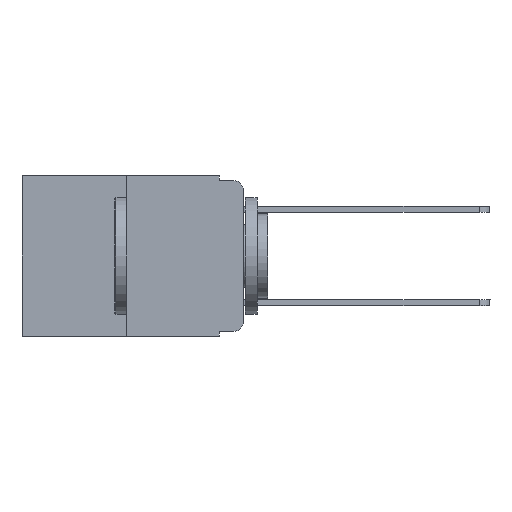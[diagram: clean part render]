
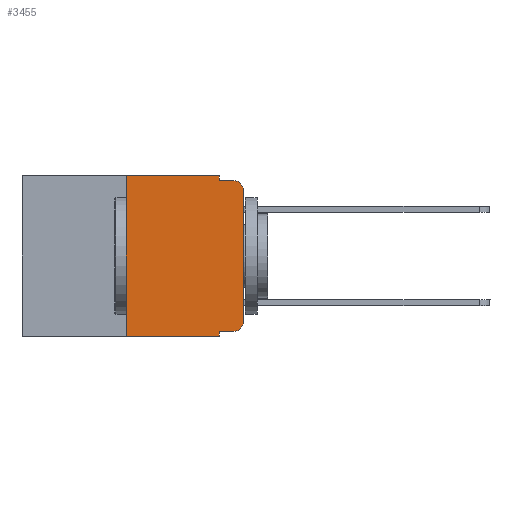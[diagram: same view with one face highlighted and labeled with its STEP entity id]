
A CAD part, left-side view. The second image highlights one B-rep face of the part: STEP entity #3455.
In plain terms, the highlighted planar face has unit normal (-1, 0, 0).
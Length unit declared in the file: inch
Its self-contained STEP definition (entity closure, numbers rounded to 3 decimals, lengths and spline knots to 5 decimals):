
#114 = VECTOR ( 'NONE', #10365, 39.37008 ) ;
#116 = ORIENTED_EDGE ( 'NONE', *, *, #11149, .F. ) ;
#227 = DIRECTION ( 'NONE',  ( 1., 0., 0. ) ) ;
#368 = CARTESIAN_POINT ( 'NONE',  ( 0., 0.473, -0.343 ) ) ;
#568 = LINE ( 'NONE', #5868, #9003 ) ;
#753 = VECTOR ( 'NONE', #10379, 39.37008 ) ;
#984 = EDGE_CURVE ( 'NONE', #3348, #5805, #3113, .T. ) ;
#985 = VERTEX_POINT ( 'NONE', #1463 ) ;
#1034 = LINE ( 'NONE', #7324, #5397 ) ;
#1243 = EDGE_CURVE ( 'NONE', #4379, #985, #5029, .T. ) ;
#1323 = CARTESIAN_POINT ( 'NONE',  ( 0., 0.02, -0.313 ) ) ;
#1440 = VECTOR ( 'NONE', #9145, 39.37008 ) ;
#1463 = CARTESIAN_POINT ( 'NONE',  ( 0., 0.051, -0.01 ) ) ;
#1708 = VECTOR ( 'NONE', #5813, 39.37008 ) ;
#1831 = VERTEX_POINT ( 'NONE', #11547 ) ;
#1904 = AXIS2_PLACEMENT_3D ( 'NONE', #4094, #11251, #4878 ) ;
#2291 = CARTESIAN_POINT ( 'NONE',  ( 0., 0.02, -0.333 ) ) ;
#2340 = ORIENTED_EDGE ( 'NONE', *, *, #6631, .T. ) ;
#2449 = EDGE_CURVE ( 'NONE', #5965, #1831, #10998, .T. ) ;
#2513 = CARTESIAN_POINT ( 'NONE',  ( 0., 0.051, 0. ) ) ;
#2537 = ORIENTED_EDGE ( 'NONE', *, *, #7189, .T. ) ;
#2625 = ORIENTED_EDGE ( 'NONE', *, *, #10282, .F. ) ;
#2882 = FACE_OUTER_BOUND ( 'NONE', #5042, .T. ) ;
#2916 = DIRECTION ( 'NONE',  ( 0., -1., 0. ) ) ;
#2950 = CARTESIAN_POINT ( 'NONE',  ( 0., 0.02, -0.01 ) ) ;
#3001 = VECTOR ( 'NONE', #6108, 39.37008 ) ;
#3113 = LINE ( 'NONE', #6673, #1708 ) ;
#3348 = VERTEX_POINT ( 'NONE', #7024 ) ;
#3455 = ADVANCED_FACE ( 'NONE', ( #2882 ), #7311, .F. ) ;
#3855 = ORIENTED_EDGE ( 'NONE', *, *, #2449, .T. ) ;
#3923 = CIRCLE ( 'NONE', #10488, 0.02 ) ;
#4005 = CARTESIAN_POINT ( 'NONE',  ( 0., 0.051, -0.343 ) ) ;
#4086 = CARTESIAN_POINT ( 'NONE',  ( 0., 0., 0. ) ) ;
#4094 = CARTESIAN_POINT ( 'NONE',  ( 0., 0.02, -0.03 ) ) ;
#4379 = VERTEX_POINT ( 'NONE', #8278 ) ;
#4878 = DIRECTION ( 'NONE',  ( 0., 0., -1. ) ) ;
#4922 = DIRECTION ( 'NONE',  ( 0., 0., -1. ) ) ;
#5029 = LINE ( 'NONE', #2513, #3001 ) ;
#5042 = EDGE_LOOP ( 'NONE', ( #3855, #2340, #2625, #10853, #8882, #116, #10168, #6618, #6602, #2537 ) ) ;
#5397 = VECTOR ( 'NONE', #8997, 39.37008 ) ;
#5497 = CARTESIAN_POINT ( 'NONE',  ( 0., 0.25, -0.343 ) ) ;
#5643 = DIRECTION ( 'NONE',  ( 0., 0., -1. ) ) ;
#5805 = VERTEX_POINT ( 'NONE', #2291 ) ;
#5813 = DIRECTION ( 'NONE',  ( 0., -1., 0. ) ) ;
#5868 = CARTESIAN_POINT ( 'NONE',  ( 0., 0.051, 0. ) ) ;
#5892 = LINE ( 'NONE', #368, #114 ) ;
#5965 = VERTEX_POINT ( 'NONE', #11501 ) ;
#6108 = DIRECTION ( 'NONE',  ( 0., 0., -1. ) ) ;
#6267 = CARTESIAN_POINT ( 'NONE',  ( 0., 0.473, 0. ) ) ;
#6296 = VERTEX_POINT ( 'NONE', #4005 ) ;
#6602 = ORIENTED_EDGE ( 'NONE', *, *, #984, .T. ) ;
#6613 = EDGE_CURVE ( 'NONE', #3348, #6296, #568, .T. ) ;
#6618 = ORIENTED_EDGE ( 'NONE', *, *, #6613, .F. ) ;
#6631 = EDGE_CURVE ( 'NONE', #1831, #11260, #8426, .T. ) ;
#6673 = CARTESIAN_POINT ( 'NONE',  ( 0., 0.051, -0.333 ) ) ;
#6729 = DIRECTION ( 'NONE',  ( 0., 0., -1. ) ) ;
#6914 = EDGE_CURVE ( 'NONE', #8554, #4379, #10088, .T. ) ;
#7015 = VERTEX_POINT ( 'NONE', #5497 ) ;
#7024 = CARTESIAN_POINT ( 'NONE',  ( 0., 0.051, -0.333 ) ) ;
#7135 = CARTESIAN_POINT ( 'NONE',  ( 0., 0.25, 0. ) ) ;
#7189 = EDGE_CURVE ( 'NONE', #5805, #5965, #3923, .T. ) ;
#7311 = PLANE ( 'NONE',  #9268 ) ;
#7324 = CARTESIAN_POINT ( 'NONE',  ( 0., 0.25, 0. ) ) ;
#7398 = CARTESIAN_POINT ( 'NONE',  ( 0., 0.473, 0. ) ) ;
#8278 = CARTESIAN_POINT ( 'NONE',  ( 0., 0.051, 0. ) ) ;
#8426 = CIRCLE ( 'NONE', #1904, 0.02 ) ;
#8554 = VERTEX_POINT ( 'NONE', #7135 ) ;
#8882 = ORIENTED_EDGE ( 'NONE', *, *, #6914, .F. ) ;
#8997 = DIRECTION ( 'NONE',  ( 0., 0., 1. ) ) ;
#9003 = VECTOR ( 'NONE', #6729, 39.37008 ) ;
#9081 = LINE ( 'NONE', #9914, #1440 ) ;
#9145 = DIRECTION ( 'NONE',  ( 0., -1., 0. ) ) ;
#9268 = AXIS2_PLACEMENT_3D ( 'NONE', #6267, #227, #5643 ) ;
#9914 = CARTESIAN_POINT ( 'NONE',  ( 0., 0.051, -0.01 ) ) ;
#10088 = LINE ( 'NONE', #7398, #10358 ) ;
#10168 = ORIENTED_EDGE ( 'NONE', *, *, #10825, .T. ) ;
#10282 = EDGE_CURVE ( 'NONE', #985, #11260, #9081, .T. ) ;
#10358 = VECTOR ( 'NONE', #2916, 39.37008 ) ;
#10365 = DIRECTION ( 'NONE',  ( 0., -1., 0. ) ) ;
#10379 = DIRECTION ( 'NONE',  ( 0., 0., 1. ) ) ;
#10488 = AXIS2_PLACEMENT_3D ( 'NONE', #1323, #11294, #4922 ) ;
#10825 = EDGE_CURVE ( 'NONE', #7015, #6296, #5892, .T. ) ;
#10853 = ORIENTED_EDGE ( 'NONE', *, *, #1243, .F. ) ;
#10998 = LINE ( 'NONE', #4086, #753 ) ;
#11149 = EDGE_CURVE ( 'NONE', #7015, #8554, #1034, .T. ) ;
#11251 = DIRECTION ( 'NONE',  ( -1., 0., 0. ) ) ;
#11260 = VERTEX_POINT ( 'NONE', #2950 ) ;
#11294 = DIRECTION ( 'NONE',  ( -1., 0., 0. ) ) ;
#11501 = CARTESIAN_POINT ( 'NONE',  ( 0., 0., -0.313 ) ) ;
#11547 = CARTESIAN_POINT ( 'NONE',  ( 0., 0., -0.03 ) ) ;
